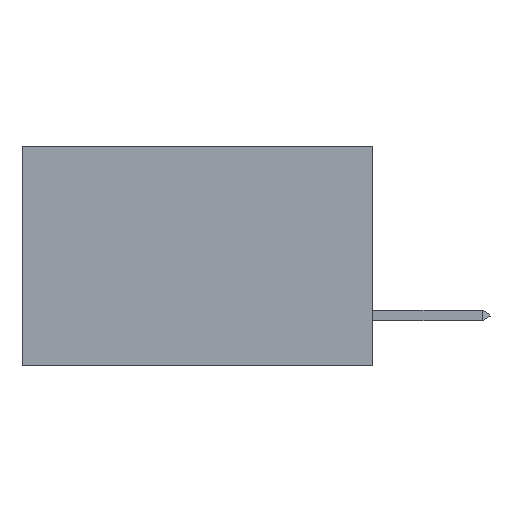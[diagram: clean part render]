
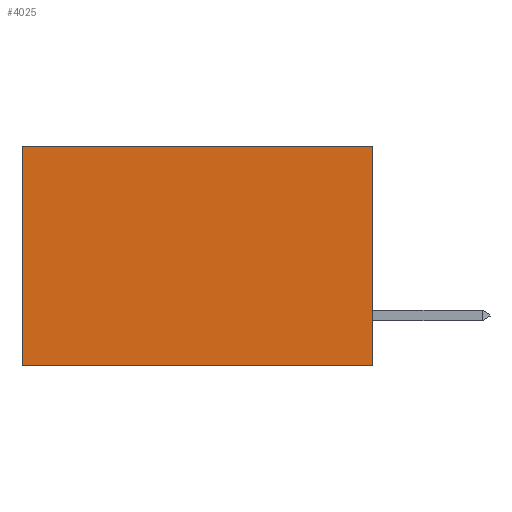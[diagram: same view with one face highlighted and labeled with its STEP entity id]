
A CAD part, left-side view. The second image highlights one B-rep face of the part: STEP entity #4025.
In plain terms, the highlighted planar face has unit normal (-1, 0, 0).
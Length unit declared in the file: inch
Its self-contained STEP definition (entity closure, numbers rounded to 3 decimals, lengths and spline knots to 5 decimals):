
#228 = VECTOR ( 'NONE', #3168, 39.37008 ) ;
#482 = EDGE_CURVE ( 'NONE', #11741, #939, #5420, .T. ) ;
#939 = VERTEX_POINT ( 'NONE', #8454 ) ;
#1734 = VECTOR ( 'NONE', #4813, 39.37008 ) ;
#1980 = EDGE_CURVE ( 'NONE', #939, #4129, #4333, .T. ) ;
#2594 = ORIENTED_EDGE ( 'NONE', *, *, #482, .T. ) ;
#3092 = CARTESIAN_POINT ( 'NONE',  ( 0.277, 0.59, -0.37 ) ) ;
#3168 = DIRECTION ( 'NONE',  ( 0., 1., 0. ) ) ;
#4025 = ADVANCED_FACE ( 'NONE', ( #4691 ), #12403, .F. ) ;
#4129 = VERTEX_POINT ( 'NONE', #11692 ) ;
#4157 = EDGE_LOOP ( 'NONE', ( #4633, #9690, #12214, #2594 ) ) ;
#4333 = LINE ( 'NONE', #3092, #9104 ) ;
#4483 = DIRECTION ( 'NONE',  ( 0., 1., 0. ) ) ;
#4633 = ORIENTED_EDGE ( 'NONE', *, *, #1980, .T. ) ;
#4691 = FACE_OUTER_BOUND ( 'NONE', #4157, .T. ) ;
#4758 = DIRECTION ( 'NONE',  ( 0., 0., -1. ) ) ;
#4813 = DIRECTION ( 'NONE',  ( 0., 0., -1. ) ) ;
#4865 = CARTESIAN_POINT ( 'NONE',  ( 0.277, 0., 0. ) ) ;
#5420 = LINE ( 'NONE', #4865, #228 ) ;
#6546 = VERTEX_POINT ( 'NONE', #7255 ) ;
#7255 = CARTESIAN_POINT ( 'NONE',  ( 0.277, 0., -0.37 ) ) ;
#8454 = CARTESIAN_POINT ( 'NONE',  ( 0.277, 0.59, 0. ) ) ;
#8810 = EDGE_CURVE ( 'NONE', #11741, #6546, #11423, .T. ) ;
#9104 = VECTOR ( 'NONE', #4758, 39.37008 ) ;
#9594 = VECTOR ( 'NONE', #4483, 39.37008 ) ;
#9690 = ORIENTED_EDGE ( 'NONE', *, *, #11316, .F. ) ;
#10624 = CARTESIAN_POINT ( 'NONE',  ( 0.277, 0., 0. ) ) ;
#11119 = CARTESIAN_POINT ( 'NONE',  ( 0.277, 0., -0.37 ) ) ;
#11316 = EDGE_CURVE ( 'NONE', #6546, #4129, #12113, .T. ) ;
#11423 = LINE ( 'NONE', #11447, #1734 ) ;
#11447 = CARTESIAN_POINT ( 'NONE',  ( 0.277, 0., -0.37 ) ) ;
#11544 = AXIS2_PLACEMENT_3D ( 'NONE', #12279, #12238, #12228 ) ;
#11692 = CARTESIAN_POINT ( 'NONE',  ( 0.277, 0.59, -0.37 ) ) ;
#11741 = VERTEX_POINT ( 'NONE', #10624 ) ;
#12113 = LINE ( 'NONE', #11119, #9594 ) ;
#12214 = ORIENTED_EDGE ( 'NONE', *, *, #8810, .F. ) ;
#12228 = DIRECTION ( 'NONE',  ( 0., 0., -1. ) ) ;
#12238 = DIRECTION ( 'NONE',  ( 1., 0., 0. ) ) ;
#12279 = CARTESIAN_POINT ( 'NONE',  ( 0.277, 0., -0.37 ) ) ;
#12403 = PLANE ( 'NONE',  #11544 ) ;
